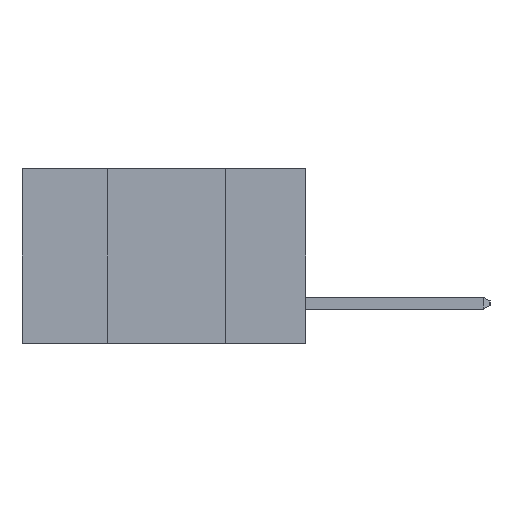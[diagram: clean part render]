
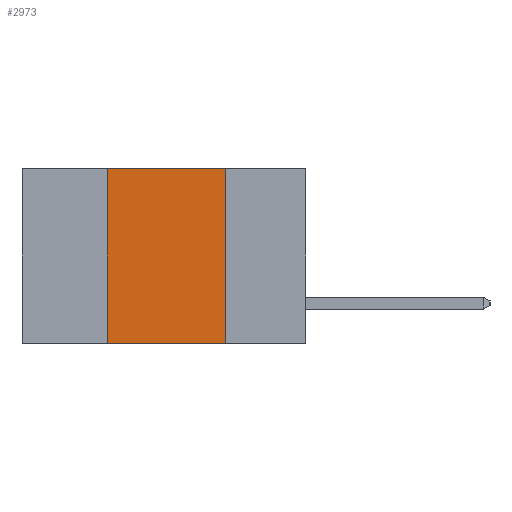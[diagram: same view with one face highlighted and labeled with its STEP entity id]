
A CAD part, left-side view. The second image highlights one B-rep face of the part: STEP entity #2973.
In plain terms, the highlighted planar face has unit normal (-1, 0, 0).
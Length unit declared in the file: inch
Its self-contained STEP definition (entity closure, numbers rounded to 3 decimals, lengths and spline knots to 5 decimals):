
#645 = DIRECTION ( 'NONE',  ( 0., -1., 0. ) ) ;
#858 = VERTEX_POINT ( 'NONE', #11158 ) ;
#1252 = LINE ( 'NONE', #11618, #8785 ) ;
#1932 = CARTESIAN_POINT ( 'NONE',  ( 0., 0.6, 0. ) ) ;
#2108 = VECTOR ( 'NONE', #12940, 39.37008 ) ;
#2300 = VECTOR ( 'NONE', #645, 39.37008 ) ;
#2862 = VERTEX_POINT ( 'NONE', #12723 ) ;
#2931 = EDGE_CURVE ( 'NONE', #2862, #4150, #6550, .T. ) ;
#2973 = ADVANCED_FACE ( 'NONE', ( #8567 ), #6194, .F. ) ;
#3647 = EDGE_CURVE ( 'NONE', #11626, #2862, #12593, .T. ) ;
#4150 = VERTEX_POINT ( 'NONE', #11794 ) ;
#4327 = EDGE_CURVE ( 'NONE', #858, #11626, #7605, .T. ) ;
#6136 = ORIENTED_EDGE ( 'NONE', *, *, #2931, .F. ) ;
#6159 = ORIENTED_EDGE ( 'NONE', *, *, #3647, .F. ) ;
#6178 = CARTESIAN_POINT ( 'NONE',  ( 0., 0.6, 0. ) ) ;
#6194 = PLANE ( 'NONE',  #7103 ) ;
#6196 = ORIENTED_EDGE ( 'NONE', *, *, #4327, .F. ) ;
#6208 = ORIENTED_EDGE ( 'NONE', *, *, #6379, .T. ) ;
#6272 = DIRECTION ( 'NONE',  ( 0., 0., -1. ) ) ;
#6330 = DIRECTION ( 'NONE',  ( 1., 0., 0. ) ) ;
#6379 = EDGE_CURVE ( 'NONE', #858, #4150, #1252, .T. ) ;
#6550 = LINE ( 'NONE', #6693, #11450 ) ;
#6693 = CARTESIAN_POINT ( 'NONE',  ( 0., 0.17, -0.37 ) ) ;
#6796 = EDGE_LOOP ( 'NONE', ( #6136, #6159, #6196, #6208 ) ) ;
#6848 = DIRECTION ( 'NONE',  ( 0., 0., -1. ) ) ;
#7103 = AXIS2_PLACEMENT_3D ( 'NONE', #6178, #6330, #6272 ) ;
#7605 = LINE ( 'NONE', #11070, #2108 ) ;
#8567 = FACE_OUTER_BOUND ( 'NONE', #6796, .T. ) ;
#8582 = CARTESIAN_POINT ( 'NONE',  ( 0., 0.42, 0. ) ) ;
#8785 = VECTOR ( 'NONE', #10646, 39.37008 ) ;
#10646 = DIRECTION ( 'NONE',  ( 0., -1., 0. ) ) ;
#11070 = CARTESIAN_POINT ( 'NONE',  ( 0., 0.42, -0.37 ) ) ;
#11158 = CARTESIAN_POINT ( 'NONE',  ( 0., 0.42, -0.37 ) ) ;
#11450 = VECTOR ( 'NONE', #6848, 39.37008 ) ;
#11618 = CARTESIAN_POINT ( 'NONE',  ( 0., 0.6, -0.37 ) ) ;
#11626 = VERTEX_POINT ( 'NONE', #8582 ) ;
#11794 = CARTESIAN_POINT ( 'NONE',  ( 0., 0.17, -0.37 ) ) ;
#12593 = LINE ( 'NONE', #1932, #2300 ) ;
#12723 = CARTESIAN_POINT ( 'NONE',  ( 0., 0.17, 0. ) ) ;
#12940 = DIRECTION ( 'NONE',  ( 0., 0., 1. ) ) ;
